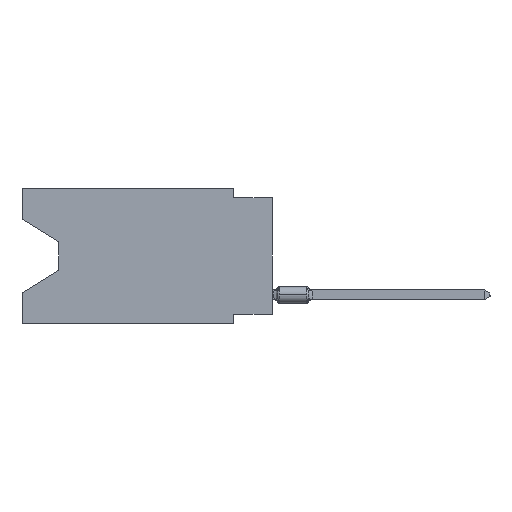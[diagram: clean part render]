
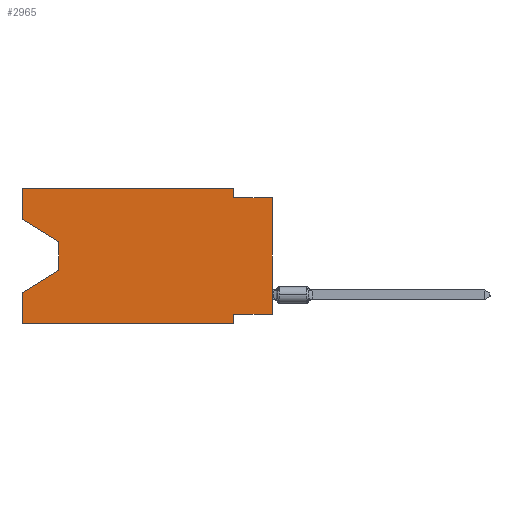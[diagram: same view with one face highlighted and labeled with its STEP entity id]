
A CAD part, left-side view. The second image highlights one B-rep face of the part: STEP entity #2965.
In plain terms, the highlighted planar face has unit normal (-1, 0, 0).
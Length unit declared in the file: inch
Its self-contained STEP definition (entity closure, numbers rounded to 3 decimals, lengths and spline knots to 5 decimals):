
#342 = VERTEX_POINT ( 'NONE', #8052 ) ;
#374 = ORIENTED_EDGE ( 'NONE', *, *, #2349, .T. ) ;
#816 = ORIENTED_EDGE ( 'NONE', *, *, #11391, .T. ) ;
#1668 = DIRECTION ( 'NONE',  ( 0., -1., 0. ) ) ;
#2069 = VECTOR ( 'NONE', #19802, 39.37008 ) ;
#2235 = VECTOR ( 'NONE', #15361, 39.37008 ) ;
#2349 = EDGE_CURVE ( 'NONE', #2882, #10148, #12002, .T. ) ;
#2631 = VECTOR ( 'NONE', #16565, 39.37008 ) ;
#2719 = EDGE_CURVE ( 'NONE', #27524, #9266, #13999, .T. ) ;
#2882 = VERTEX_POINT ( 'NONE', #9748 ) ;
#2965 = ADVANCED_FACE ( 'NONE', ( #26677 ), #13125, .F. ) ;
#4270 = VECTOR ( 'NONE', #1668, 39.37008 ) ;
#4484 = CARTESIAN_POINT ( 'NONE',  ( 0., 0.1, -0.35 ) ) ;
#4977 = DIRECTION ( 'NONE',  ( 0., -1., 0. ) ) ;
#5393 = CARTESIAN_POINT ( 'NONE',  ( 0., 0.645, 0. ) ) ;
#6069 = ORIENTED_EDGE ( 'NONE', *, *, #23054, .F. ) ;
#6169 = CARTESIAN_POINT ( 'NONE',  ( 0., 0.1, 0. ) ) ;
#7198 = CARTESIAN_POINT ( 'NONE',  ( 0., 0., 0. ) ) ;
#7297 = EDGE_CURVE ( 'NONE', #342, #24133, #26440, .T. ) ;
#7459 = ORIENTED_EDGE ( 'NONE', *, *, #2719, .F. ) ;
#7525 = LINE ( 'NONE', #7198, #2235 ) ;
#7800 = CARTESIAN_POINT ( 'NONE',  ( 0., 0.1, -0.325 ) ) ;
#7810 = CARTESIAN_POINT ( 'NONE',  ( 0., 0.1, 0. ) ) ;
#8052 = CARTESIAN_POINT ( 'NONE',  ( 0., 0.645, -0.35 ) ) ;
#8146 = ORIENTED_EDGE ( 'NONE', *, *, #7297, .F. ) ;
#8202 = CARTESIAN_POINT ( 'NONE',  ( 0., 0.645, -0.26975 ) ) ;
#8368 = VERTEX_POINT ( 'NONE', #7800 ) ;
#8460 = DIRECTION ( 'NONE',  ( 0., 0., 1. ) ) ;
#9096 = CARTESIAN_POINT ( 'NONE',  ( 0., 0.55, -0.212 ) ) ;
#9230 = VERTEX_POINT ( 'NONE', #13967 ) ;
#9266 = VERTEX_POINT ( 'NONE', #31452 ) ;
#9275 = CARTESIAN_POINT ( 'NONE',  ( 0., 0., -0.025 ) ) ;
#9331 = EDGE_CURVE ( 'NONE', #342, #31318, #10020, .T. ) ;
#9556 = EDGE_CURVE ( 'NONE', #2882, #27965, #23229, .T. ) ;
#9657 = CARTESIAN_POINT ( 'NONE',  ( 0., 0.645, 0. ) ) ;
#9748 = CARTESIAN_POINT ( 'NONE',  ( 0., 0.645, -0.08025 ) ) ;
#10020 = LINE ( 'NONE', #27820, #4270 ) ;
#10117 = DIRECTION ( 'NONE',  ( 0., 0., -1. ) ) ;
#10148 = VERTEX_POINT ( 'NONE', #19937 ) ;
#10287 = CARTESIAN_POINT ( 'NONE',  ( 0., 0., -0.325 ) ) ;
#10364 = VECTOR ( 'NONE', #20630, 39.37008 ) ;
#10747 = DIRECTION ( 'NONE',  ( 0., 0., -1. ) ) ;
#11391 = EDGE_CURVE ( 'NONE', #30951, #24133, #31834, .T. ) ;
#11962 = DIRECTION ( 'NONE',  ( 0., 0., -1. ) ) ;
#12002 = LINE ( 'NONE', #14208, #2069 ) ;
#13038 = LINE ( 'NONE', #28306, #28356 ) ;
#13095 = VECTOR ( 'NONE', #19863, 39.37008 ) ;
#13125 = PLANE ( 'NONE',  #20000 ) ;
#13294 = CARTESIAN_POINT ( 'NONE',  ( 0., 0.645, 0. ) ) ;
#13911 = ORIENTED_EDGE ( 'NONE', *, *, #18344, .T. ) ;
#13967 = CARTESIAN_POINT ( 'NONE',  ( 0., 0., -0.325 ) ) ;
#13999 = LINE ( 'NONE', #6169, #19464 ) ;
#14208 = CARTESIAN_POINT ( 'NONE',  ( 0., 0.645, -0.08025 ) ) ;
#15361 = DIRECTION ( 'NONE',  ( 0., 0., 1. ) ) ;
#16142 = EDGE_LOOP ( 'NONE', ( #374, #13911, #816, #8146, #29498, #23364, #31487, #20195, #6069, #7459, #33001, #19129 ) ) ;
#16565 = DIRECTION ( 'NONE',  ( 0., 0.855, -0.519 ) ) ;
#17033 = VECTOR ( 'NONE', #10117, 39.37008 ) ;
#18344 = EDGE_CURVE ( 'NONE', #10148, #30951, #13038, .T. ) ;
#19129 = ORIENTED_EDGE ( 'NONE', *, *, #9556, .F. ) ;
#19464 = VECTOR ( 'NONE', #11962, 39.37008 ) ;
#19802 = DIRECTION ( 'NONE',  ( 0., -0.855, -0.519 ) ) ;
#19863 = DIRECTION ( 'NONE',  ( 0., -1., 0. ) ) ;
#19937 = CARTESIAN_POINT ( 'NONE',  ( 0., 0.55, -0.138 ) ) ;
#20000 = AXIS2_PLACEMENT_3D ( 'NONE', #13294, #31114, #10747 ) ;
#20195 = ORIENTED_EDGE ( 'NONE', *, *, #22811, .T. ) ;
#20630 = DIRECTION ( 'NONE',  ( 0., 1., 0. ) ) ;
#22486 = EDGE_CURVE ( 'NONE', #9230, #8368, #25728, .T. ) ;
#22807 = EDGE_CURVE ( 'NONE', #27965, #27524, #23153, .T. ) ;
#22811 = EDGE_CURVE ( 'NONE', #9230, #26987, #7525, .T. ) ;
#23054 = EDGE_CURVE ( 'NONE', #9266, #26987, #32591, .T. ) ;
#23153 = LINE ( 'NONE', #32842, #31532 ) ;
#23229 = LINE ( 'NONE', #31542, #27028 ) ;
#23364 = ORIENTED_EDGE ( 'NONE', *, *, #30884, .F. ) ;
#23743 = CARTESIAN_POINT ( 'NONE',  ( 0., 0.1, -0.35 ) ) ;
#24133 = VERTEX_POINT ( 'NONE', #8202 ) ;
#25610 = DIRECTION ( 'NONE',  ( 0., 0., 1. ) ) ;
#25728 = LINE ( 'NONE', #10287, #10364 ) ;
#26096 = DIRECTION ( 'NONE',  ( 0., 0., -1. ) ) ;
#26440 = LINE ( 'NONE', #5393, #29201 ) ;
#26677 = FACE_OUTER_BOUND ( 'NONE', #16142, .T. ) ;
#26987 = VERTEX_POINT ( 'NONE', #9275 ) ;
#27028 = VECTOR ( 'NONE', #25610, 39.37008 ) ;
#27524 = VERTEX_POINT ( 'NONE', #7810 ) ;
#27749 = LINE ( 'NONE', #4484, #17033 ) ;
#27820 = CARTESIAN_POINT ( 'NONE',  ( 0., 0.645, -0.35 ) ) ;
#27965 = VERTEX_POINT ( 'NONE', #9657 ) ;
#28306 = CARTESIAN_POINT ( 'NONE',  ( 0., 0.55, -0.138 ) ) ;
#28356 = VECTOR ( 'NONE', #26096, 39.37008 ) ;
#29201 = VECTOR ( 'NONE', #8460, 39.37008 ) ;
#29498 = ORIENTED_EDGE ( 'NONE', *, *, #9331, .T. ) ;
#30884 = EDGE_CURVE ( 'NONE', #8368, #31318, #27749, .T. ) ;
#30951 = VERTEX_POINT ( 'NONE', #30972 ) ;
#30972 = CARTESIAN_POINT ( 'NONE',  ( 0., 0.55, -0.212 ) ) ;
#31114 = DIRECTION ( 'NONE',  ( 1., 0., 0. ) ) ;
#31318 = VERTEX_POINT ( 'NONE', #23743 ) ;
#31452 = CARTESIAN_POINT ( 'NONE',  ( 0., 0.1, -0.025 ) ) ;
#31487 = ORIENTED_EDGE ( 'NONE', *, *, #22486, .F. ) ;
#31532 = VECTOR ( 'NONE', #4977, 39.37008 ) ;
#31542 = CARTESIAN_POINT ( 'NONE',  ( 0., 0.645, 0. ) ) ;
#31834 = LINE ( 'NONE', #9096, #2631 ) ;
#32416 = CARTESIAN_POINT ( 'NONE',  ( 0., 0., -0.025 ) ) ;
#32591 = LINE ( 'NONE', #32416, #13095 ) ;
#32842 = CARTESIAN_POINT ( 'NONE',  ( 0., 0.645, 0. ) ) ;
#33001 = ORIENTED_EDGE ( 'NONE', *, *, #22807, .F. ) ;
